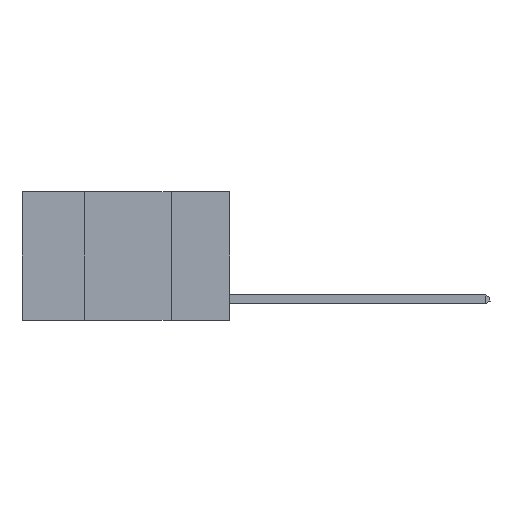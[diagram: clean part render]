
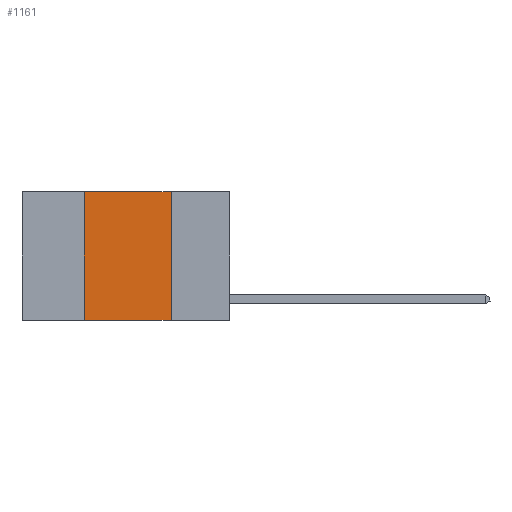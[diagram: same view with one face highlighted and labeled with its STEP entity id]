
A CAD part, left-side view. The second image highlights one B-rep face of the part: STEP entity #1161.
In plain terms, the highlighted planar face has unit normal (-1, 0, 0).
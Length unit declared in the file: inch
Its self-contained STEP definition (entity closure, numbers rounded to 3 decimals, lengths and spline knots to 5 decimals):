
#29 = CARTESIAN_POINT ( 'NONE',  ( 0., 0.6, 0. ) ) ;
#370 = EDGE_CURVE ( 'NONE', #9359, #2092, #7034, .T. ) ;
#523 = CARTESIAN_POINT ( 'NONE',  ( 0., 0.42, 0. ) ) ;
#660 = DIRECTION ( 'NONE',  ( 0., 0., -1. ) ) ;
#826 = VECTOR ( 'NONE', #7128, 39.37008 ) ;
#1161 = ADVANCED_FACE ( 'NONE', ( #3731 ), #6720, .F. ) ;
#1526 = VECTOR ( 'NONE', #8323, 39.37008 ) ;
#2078 = ORIENTED_EDGE ( 'NONE', *, *, #5066, .F. ) ;
#2092 = VERTEX_POINT ( 'NONE', #6057 ) ;
#2253 = CARTESIAN_POINT ( 'NONE',  ( 0., 0.17, 0. ) ) ;
#2529 = ORIENTED_EDGE ( 'NONE', *, *, #7981, .F. ) ;
#3165 = CARTESIAN_POINT ( 'NONE',  ( 0., 0.6, 0. ) ) ;
#3396 = DIRECTION ( 'NONE',  ( 0., 0., 1. ) ) ;
#3495 = LINE ( 'NONE', #523, #8083 ) ;
#3566 = CARTESIAN_POINT ( 'NONE',  ( 0., 0.42, 0. ) ) ;
#3731 = FACE_OUTER_BOUND ( 'NONE', #5081, .T. ) ;
#3873 = DIRECTION ( 'NONE',  ( 0., 0., -1. ) ) ;
#4614 = LINE ( 'NONE', #3165, #1526 ) ;
#4963 = AXIS2_PLACEMENT_3D ( 'NONE', #29, #8951, #660 ) ;
#5066 = EDGE_CURVE ( 'NONE', #9359, #6975, #3495, .T. ) ;
#5081 = EDGE_LOOP ( 'NONE', ( #6193, #2529, #2078, #6172 ) ) ;
#5194 = CARTESIAN_POINT ( 'NONE',  ( 0., 0.42, -0.37 ) ) ;
#6057 = CARTESIAN_POINT ( 'NONE',  ( 0., 0.17, -0.37 ) ) ;
#6172 = ORIENTED_EDGE ( 'NONE', *, *, #370, .T. ) ;
#6193 = ORIENTED_EDGE ( 'NONE', *, *, #6596, .F. ) ;
#6596 = EDGE_CURVE ( 'NONE', #9393, #2092, #6806, .T. ) ;
#6720 = PLANE ( 'NONE',  #4963 ) ;
#6806 = LINE ( 'NONE', #8945, #8273 ) ;
#6975 = VERTEX_POINT ( 'NONE', #3566 ) ;
#7034 = LINE ( 'NONE', #9264, #826 ) ;
#7128 = DIRECTION ( 'NONE',  ( 0., -1., 0. ) ) ;
#7981 = EDGE_CURVE ( 'NONE', #6975, #9393, #4614, .T. ) ;
#8083 = VECTOR ( 'NONE', #3396, 39.37008 ) ;
#8273 = VECTOR ( 'NONE', #3873, 39.37008 ) ;
#8323 = DIRECTION ( 'NONE',  ( 0., -1., 0. ) ) ;
#8945 = CARTESIAN_POINT ( 'NONE',  ( 0., 0.17, 0. ) ) ;
#8951 = DIRECTION ( 'NONE',  ( 1., 0., 0. ) ) ;
#9264 = CARTESIAN_POINT ( 'NONE',  ( 0., 0.6, -0.37 ) ) ;
#9359 = VERTEX_POINT ( 'NONE', #5194 ) ;
#9393 = VERTEX_POINT ( 'NONE', #2253 ) ;
